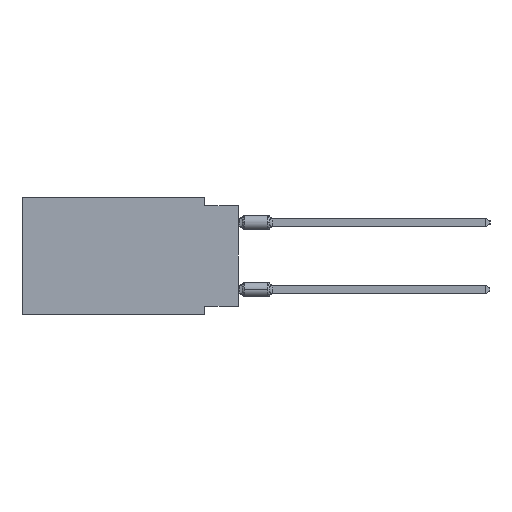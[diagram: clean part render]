
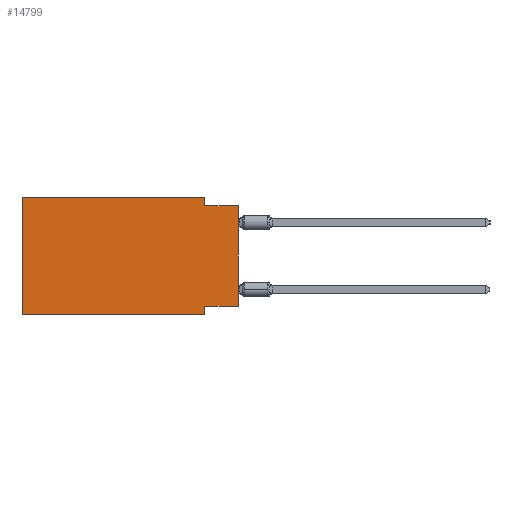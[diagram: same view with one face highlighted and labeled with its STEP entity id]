
A CAD part, left-side view. The second image highlights one B-rep face of the part: STEP entity #14799.
In plain terms, the highlighted planar face has unit normal (-1, 0, 0).
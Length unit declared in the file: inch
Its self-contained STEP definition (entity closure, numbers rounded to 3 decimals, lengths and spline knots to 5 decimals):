
#225 = CARTESIAN_POINT ( 'NONE',  ( 0., 0., -0.025 ) ) ;
#534 = CARTESIAN_POINT ( 'NONE',  ( 0., 0.1, 0. ) ) ;
#2997 = LINE ( 'NONE', #38009, #26515 ) ;
#3076 = ORIENTED_EDGE ( 'NONE', *, *, #48571, .F. ) ;
#3156 = CARTESIAN_POINT ( 'NONE',  ( 0., 0.645, -0.35 ) ) ;
#3849 = DIRECTION ( 'NONE',  ( 0., 1., 0. ) ) ;
#7238 = DIRECTION ( 'NONE',  ( 1., 0., 0. ) ) ;
#7806 = EDGE_CURVE ( 'NONE', #16927, #34553, #13106, .T. ) ;
#8574 = ORIENTED_EDGE ( 'NONE', *, *, #22235, .T. ) ;
#8736 = ORIENTED_EDGE ( 'NONE', *, *, #32439, .F. ) ;
#10333 = EDGE_CURVE ( 'NONE', #35037, #16927, #13221, .T. ) ;
#10457 = CARTESIAN_POINT ( 'NONE',  ( 0., 0., -0.325 ) ) ;
#10683 = VECTOR ( 'NONE', #3849, 39.37008 ) ;
#10935 = PLANE ( 'NONE',  #19205 ) ;
#11484 = FACE_OUTER_BOUND ( 'NONE', #28310, .T. ) ;
#11956 = VECTOR ( 'NONE', #41272, 39.37008 ) ;
#12394 = LINE ( 'NONE', #46873, #16043 ) ;
#13106 = LINE ( 'NONE', #46085, #11956 ) ;
#13221 = LINE ( 'NONE', #55382, #10683 ) ;
#14799 = ADVANCED_FACE ( 'NONE', ( #11484 ), #10935, .F. ) ;
#16043 = VECTOR ( 'NONE', #29761, 39.37008 ) ;
#16435 = CARTESIAN_POINT ( 'NONE',  ( 0., 0.1, -0.025 ) ) ;
#16927 = VERTEX_POINT ( 'NONE', #36238 ) ;
#18852 = EDGE_CURVE ( 'NONE', #20369, #27088, #51661, .T. ) ;
#19205 = AXIS2_PLACEMENT_3D ( 'NONE', #28309, #7238, #51089 ) ;
#19746 = DIRECTION ( 'NONE',  ( 0., 0., 1. ) ) ;
#20369 = VERTEX_POINT ( 'NONE', #534 ) ;
#21864 = CARTESIAN_POINT ( 'NONE',  ( 0., 0.645, -0.35 ) ) ;
#22235 = EDGE_CURVE ( 'NONE', #39856, #34553, #37903, .T. ) ;
#26080 = VECTOR ( 'NONE', #52055, 39.37008 ) ;
#26308 = EDGE_CURVE ( 'NONE', #35037, #42354, #2997, .T. ) ;
#26515 = VECTOR ( 'NONE', #50525, 39.37008 ) ;
#27088 = VERTEX_POINT ( 'NONE', #16435 ) ;
#28309 = CARTESIAN_POINT ( 'NONE',  ( 0., 0.645, 0. ) ) ;
#28310 = EDGE_LOOP ( 'NONE', ( #48613, #3076, #29520, #34844, #8736, #8574, #32805, #40860 ) ) ;
#29520 = ORIENTED_EDGE ( 'NONE', *, *, #18852, .F. ) ;
#29761 = DIRECTION ( 'NONE',  ( 0., -1., 0. ) ) ;
#30494 = VERTEX_POINT ( 'NONE', #53193 ) ;
#32439 = EDGE_CURVE ( 'NONE', #39856, #30494, #40323, .T. ) ;
#32805 = ORIENTED_EDGE ( 'NONE', *, *, #7806, .F. ) ;
#33462 = DIRECTION ( 'NONE',  ( 0., 0., -1. ) ) ;
#34553 = VERTEX_POINT ( 'NONE', #37007 ) ;
#34844 = ORIENTED_EDGE ( 'NONE', *, *, #41628, .F. ) ;
#35037 = VERTEX_POINT ( 'NONE', #10457 ) ;
#36238 = CARTESIAN_POINT ( 'NONE',  ( 0., 0.1, -0.325 ) ) ;
#36985 = CARTESIAN_POINT ( 'NONE',  ( 0., 0., -0.025 ) ) ;
#37007 = CARTESIAN_POINT ( 'NONE',  ( 0., 0.1, -0.35 ) ) ;
#37903 = LINE ( 'NONE', #3156, #49964 ) ;
#38009 = CARTESIAN_POINT ( 'NONE',  ( 0., 0., 0. ) ) ;
#39856 = VERTEX_POINT ( 'NONE', #21864 ) ;
#40323 = LINE ( 'NONE', #49679, #47068 ) ;
#40860 = ORIENTED_EDGE ( 'NONE', *, *, #10333, .F. ) ;
#41272 = DIRECTION ( 'NONE',  ( 0., 0., -1. ) ) ;
#41628 = EDGE_CURVE ( 'NONE', #30494, #20369, #12394, .T. ) ;
#42354 = VERTEX_POINT ( 'NONE', #36985 ) ;
#43239 = LINE ( 'NONE', #225, #26080 ) ;
#46085 = CARTESIAN_POINT ( 'NONE',  ( 0., 0.1, -0.35 ) ) ;
#46873 = CARTESIAN_POINT ( 'NONE',  ( 0., 0.645, 0. ) ) ;
#47068 = VECTOR ( 'NONE', #19746, 39.37008 ) ;
#48514 = VECTOR ( 'NONE', #33462, 39.37008 ) ;
#48571 = EDGE_CURVE ( 'NONE', #27088, #42354, #43239, .T. ) ;
#48613 = ORIENTED_EDGE ( 'NONE', *, *, #26308, .T. ) ;
#49679 = CARTESIAN_POINT ( 'NONE',  ( 0., 0.645, 0. ) ) ;
#49964 = VECTOR ( 'NONE', #56090, 39.37008 ) ;
#50525 = DIRECTION ( 'NONE',  ( 0., 0., 1. ) ) ;
#50825 = CARTESIAN_POINT ( 'NONE',  ( 0., 0.1, 0. ) ) ;
#51089 = DIRECTION ( 'NONE',  ( 0., 0., -1. ) ) ;
#51661 = LINE ( 'NONE', #50825, #48514 ) ;
#52055 = DIRECTION ( 'NONE',  ( 0., -1., 0. ) ) ;
#53193 = CARTESIAN_POINT ( 'NONE',  ( 0., 0.645, 0. ) ) ;
#55382 = CARTESIAN_POINT ( 'NONE',  ( 0., 0., -0.325 ) ) ;
#56090 = DIRECTION ( 'NONE',  ( 0., -1., 0. ) ) ;
